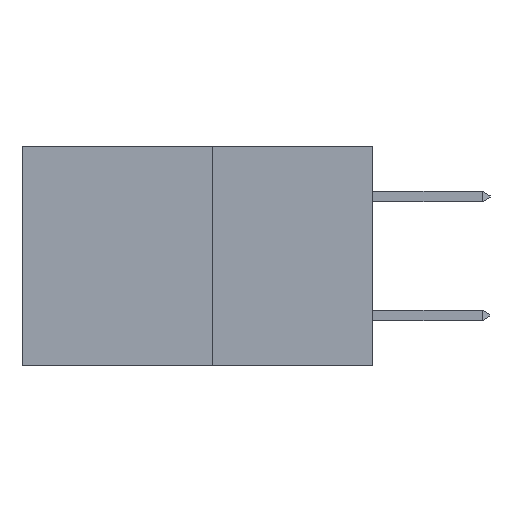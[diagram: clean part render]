
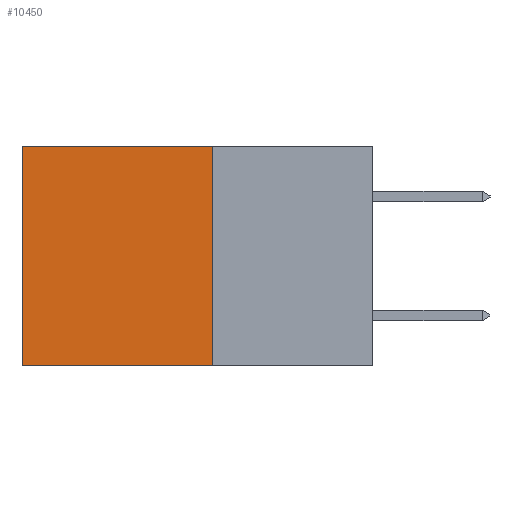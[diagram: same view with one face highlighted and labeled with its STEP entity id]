
A CAD part, left-side view. The second image highlights one B-rep face of the part: STEP entity #10450.
In plain terms, the highlighted planar face has unit normal (-1, 0, 0).
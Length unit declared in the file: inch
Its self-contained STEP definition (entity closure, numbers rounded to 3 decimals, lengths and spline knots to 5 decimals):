
#425 = DIRECTION ( 'NONE',  ( 0., 0., -1. ) ) ;
#1614 = EDGE_CURVE ( 'NONE', #10551, #8370, #9176, .T. ) ;
#1985 = AXIS2_PLACEMENT_3D ( 'NONE', #15641, #8186, #425 ) ;
#2649 = LINE ( 'NONE', #3625, #12378 ) ;
#3272 = DIRECTION ( 'NONE',  ( 0., 0., -1. ) ) ;
#3612 = DIRECTION ( 'NONE',  ( 0., 1., 0. ) ) ;
#3625 = CARTESIAN_POINT ( 'NONE',  ( 0.277, 0.27, 0. ) ) ;
#4401 = CARTESIAN_POINT ( 'NONE',  ( 0.277, 0.59, -0.37 ) ) ;
#4553 = CARTESIAN_POINT ( 'NONE',  ( 0.277, 0.27, -0.37 ) ) ;
#4898 = FACE_OUTER_BOUND ( 'NONE', #6157, .T. ) ;
#5354 = EDGE_CURVE ( 'NONE', #12536, #8370, #13001, .T. ) ;
#5530 = DIRECTION ( 'NONE',  ( 0., 1., 0. ) ) ;
#5577 = EDGE_CURVE ( 'NONE', #6095, #12536, #2649, .T. ) ;
#5581 = CARTESIAN_POINT ( 'NONE',  ( 0.277, 0.59, -0.37 ) ) ;
#5612 = PLANE ( 'NONE',  #1985 ) ;
#5747 = VECTOR ( 'NONE', #5530, 39.37008 ) ;
#5899 = CARTESIAN_POINT ( 'NONE',  ( 0.277, 0.59, 0. ) ) ;
#5913 = EDGE_CURVE ( 'NONE', #6095, #10551, #10965, .T. ) ;
#6095 = VERTEX_POINT ( 'NONE', #9796 ) ;
#6157 = EDGE_LOOP ( 'NONE', ( #11557, #10284, #13682, #8242 ) ) ;
#7628 = VECTOR ( 'NONE', #15524, 39.37008 ) ;
#8186 = DIRECTION ( 'NONE',  ( 1., 0., 0. ) ) ;
#8242 = ORIENTED_EDGE ( 'NONE', *, *, #5577, .T. ) ;
#8370 = VERTEX_POINT ( 'NONE', #5581 ) ;
#9176 = LINE ( 'NONE', #14366, #5747 ) ;
#9796 = CARTESIAN_POINT ( 'NONE',  ( 0.277, 0.27, 0. ) ) ;
#10284 = ORIENTED_EDGE ( 'NONE', *, *, #1614, .F. ) ;
#10450 = ADVANCED_FACE ( 'NONE', ( #4898 ), #5612, .F. ) ;
#10551 = VERTEX_POINT ( 'NONE', #4553 ) ;
#10965 = LINE ( 'NONE', #16136, #7628 ) ;
#11557 = ORIENTED_EDGE ( 'NONE', *, *, #5354, .T. ) ;
#12378 = VECTOR ( 'NONE', #3612, 39.37008 ) ;
#12536 = VERTEX_POINT ( 'NONE', #5899 ) ;
#13001 = LINE ( 'NONE', #4401, #15456 ) ;
#13682 = ORIENTED_EDGE ( 'NONE', *, *, #5913, .F. ) ;
#14366 = CARTESIAN_POINT ( 'NONE',  ( 0.277, 0.27, -0.37 ) ) ;
#15456 = VECTOR ( 'NONE', #3272, 39.37008 ) ;
#15524 = DIRECTION ( 'NONE',  ( 0., 0., -1. ) ) ;
#15641 = CARTESIAN_POINT ( 'NONE',  ( 0.277, 0.27, -0.37 ) ) ;
#16136 = CARTESIAN_POINT ( 'NONE',  ( 0.277, 0.27, -0.37 ) ) ;
